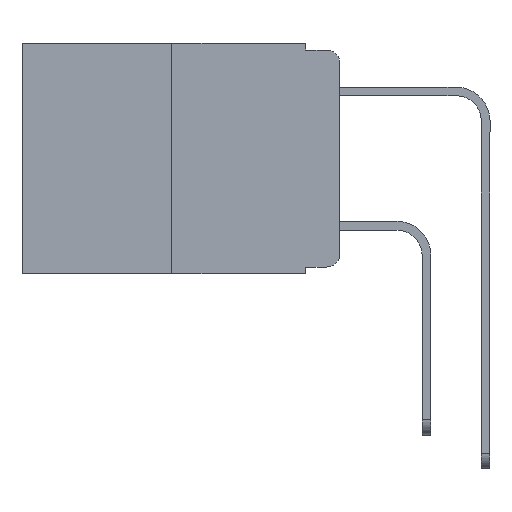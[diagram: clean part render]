
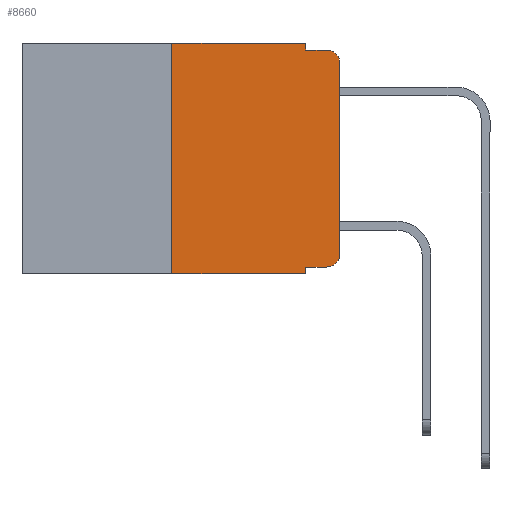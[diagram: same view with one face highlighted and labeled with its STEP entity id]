
A CAD part, left-side view. The second image highlights one B-rep face of the part: STEP entity #8660.
In plain terms, the highlighted planar face has unit normal (-1, 0, 0).
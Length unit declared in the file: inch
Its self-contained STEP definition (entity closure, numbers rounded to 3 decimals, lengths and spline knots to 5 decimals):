
#470 = CARTESIAN_POINT ( 'NONE',  ( 0., 0.25, -0.343 ) ) ;
#684 = EDGE_CURVE ( 'NONE', #8205, #2565, #3473, .T. ) ;
#721 = ORIENTED_EDGE ( 'NONE', *, *, #5792, .T. ) ;
#991 = CARTESIAN_POINT ( 'NONE',  ( 0., 0.02, -0.313 ) ) ;
#1325 = CARTESIAN_POINT ( 'NONE',  ( 0., 0.02, -0.333 ) ) ;
#1469 = CARTESIAN_POINT ( 'NONE',  ( 0., 0.051, -0.01 ) ) ;
#1771 = DIRECTION ( 'NONE',  ( 0., -1., 0. ) ) ;
#1795 = VERTEX_POINT ( 'NONE', #5593 ) ;
#1982 = DIRECTION ( 'NONE',  ( 0., 0., -1. ) ) ;
#2019 = CARTESIAN_POINT ( 'NONE',  ( 0., 0.051, -0.333 ) ) ;
#2071 = DIRECTION ( 'NONE',  ( 0., 0., -1. ) ) ;
#2134 = PLANE ( 'NONE',  #7702 ) ;
#2445 = VECTOR ( 'NONE', #9640, 39.37008 ) ;
#2565 = VERTEX_POINT ( 'NONE', #9895 ) ;
#2645 = CARTESIAN_POINT ( 'NONE',  ( 0., 0., 0. ) ) ;
#2825 = AXIS2_PLACEMENT_3D ( 'NONE', #991, #7983, #1982 ) ;
#2948 = CARTESIAN_POINT ( 'NONE',  ( 0., 0.051, 0. ) ) ;
#3001 = CARTESIAN_POINT ( 'NONE',  ( 0., 0.25, 0. ) ) ;
#3167 = CARTESIAN_POINT ( 'NONE',  ( 0., 0.473, 0. ) ) ;
#3342 = EDGE_CURVE ( 'NONE', #6581, #3847, #6236, .T. ) ;
#3381 = VECTOR ( 'NONE', #4839, 39.37008 ) ;
#3427 = CIRCLE ( 'NONE', #2825, 0.02 ) ;
#3468 = CARTESIAN_POINT ( 'NONE',  ( 0., 0.051, -0.343 ) ) ;
#3473 = LINE ( 'NONE', #1469, #11051 ) ;
#3650 = VERTEX_POINT ( 'NONE', #1325 ) ;
#3667 = EDGE_CURVE ( 'NONE', #11853, #3847, #5440, .T. ) ;
#3695 = VECTOR ( 'NONE', #6827, 39.37008 ) ;
#3847 = VERTEX_POINT ( 'NONE', #3468 ) ;
#3857 = CARTESIAN_POINT ( 'NONE',  ( 0., 0.473, 0. ) ) ;
#3896 = VECTOR ( 'NONE', #7410, 39.37008 ) ;
#3997 = DIRECTION ( 'NONE',  ( 0., 0., 1. ) ) ;
#4024 = FACE_OUTER_BOUND ( 'NONE', #6497, .T. ) ;
#4115 = AXIS2_PLACEMENT_3D ( 'NONE', #12008, #12005, #11989 ) ;
#4173 = DIRECTION ( 'NONE',  ( 0., 0., -1. ) ) ;
#4216 = EDGE_CURVE ( 'NONE', #1795, #4227, #9464, .T. ) ;
#4227 = VERTEX_POINT ( 'NONE', #10710 ) ;
#4302 = CARTESIAN_POINT ( 'NONE',  ( 0., 0.25, 0. ) ) ;
#4498 = ORIENTED_EDGE ( 'NONE', *, *, #11613, .F. ) ;
#4792 = CARTESIAN_POINT ( 'NONE',  ( 0., 0.051, -0.333 ) ) ;
#4839 = DIRECTION ( 'NONE',  ( 0., -1., 0. ) ) ;
#5440 = LINE ( 'NONE', #7324, #2445 ) ;
#5535 = EDGE_CURVE ( 'NONE', #11853, #10641, #12525, .T. ) ;
#5593 = CARTESIAN_POINT ( 'NONE',  ( 0., 0., -0.313 ) ) ;
#5792 = EDGE_CURVE ( 'NONE', #4227, #2565, #11491, .T. ) ;
#6236 = LINE ( 'NONE', #7432, #3896 ) ;
#6245 = ORIENTED_EDGE ( 'NONE', *, *, #684, .F. ) ;
#6497 = EDGE_LOOP ( 'NONE', ( #7029, #721, #6245, #4498, #12639, #8747, #10451, #9523, #11330, #8424 ) ) ;
#6581 = VERTEX_POINT ( 'NONE', #2019 ) ;
#6658 = LINE ( 'NONE', #4792, #3695 ) ;
#6827 = DIRECTION ( 'NONE',  ( 0., -1., 0. ) ) ;
#6981 = LINE ( 'NONE', #3857, #3381 ) ;
#7029 = ORIENTED_EDGE ( 'NONE', *, *, #4216, .T. ) ;
#7324 = CARTESIAN_POINT ( 'NONE',  ( 0., 0.473, -0.343 ) ) ;
#7410 = DIRECTION ( 'NONE',  ( 0., 0., -1. ) ) ;
#7415 = CARTESIAN_POINT ( 'NONE',  ( 0., 0.051, -0.01 ) ) ;
#7432 = CARTESIAN_POINT ( 'NONE',  ( 0., 0.051, 0. ) ) ;
#7702 = AXIS2_PLACEMENT_3D ( 'NONE', #3167, #10120, #4173 ) ;
#7918 = EDGE_CURVE ( 'NONE', #3650, #1795, #3427, .T. ) ;
#7983 = DIRECTION ( 'NONE',  ( -1., 0., 0. ) ) ;
#8069 = CARTESIAN_POINT ( 'NONE',  ( 0., 0.051, 0. ) ) ;
#8205 = VERTEX_POINT ( 'NONE', #7415 ) ;
#8424 = ORIENTED_EDGE ( 'NONE', *, *, #7918, .T. ) ;
#8589 = DIRECTION ( 'NONE',  ( 0., 0., 1. ) ) ;
#8660 = ADVANCED_FACE ( 'NONE', ( #4024 ), #2134, .F. ) ;
#8747 = ORIENTED_EDGE ( 'NONE', *, *, #5535, .F. ) ;
#8989 = LINE ( 'NONE', #8069, #11252 ) ;
#9464 = LINE ( 'NONE', #2645, #12007 ) ;
#9523 = ORIENTED_EDGE ( 'NONE', *, *, #3342, .F. ) ;
#9585 = EDGE_CURVE ( 'NONE', #6581, #3650, #6658, .T. ) ;
#9607 = EDGE_CURVE ( 'NONE', #10641, #11546, #6981, .T. ) ;
#9640 = DIRECTION ( 'NONE',  ( 0., -1., 0. ) ) ;
#9895 = CARTESIAN_POINT ( 'NONE',  ( 0., 0.02, -0.01 ) ) ;
#10021 = VECTOR ( 'NONE', #8589, 39.37008 ) ;
#10120 = DIRECTION ( 'NONE',  ( 1., 0., 0. ) ) ;
#10451 = ORIENTED_EDGE ( 'NONE', *, *, #3667, .T. ) ;
#10641 = VERTEX_POINT ( 'NONE', #4302 ) ;
#10710 = CARTESIAN_POINT ( 'NONE',  ( 0., 0., -0.03 ) ) ;
#11051 = VECTOR ( 'NONE', #1771, 39.37008 ) ;
#11252 = VECTOR ( 'NONE', #2071, 39.37008 ) ;
#11330 = ORIENTED_EDGE ( 'NONE', *, *, #9585, .T. ) ;
#11491 = CIRCLE ( 'NONE', #4115, 0.02 ) ;
#11546 = VERTEX_POINT ( 'NONE', #2948 ) ;
#11613 = EDGE_CURVE ( 'NONE', #11546, #8205, #8989, .T. ) ;
#11853 = VERTEX_POINT ( 'NONE', #470 ) ;
#11989 = DIRECTION ( 'NONE',  ( 0., 0., -1. ) ) ;
#12005 = DIRECTION ( 'NONE',  ( -1., 0., 0. ) ) ;
#12007 = VECTOR ( 'NONE', #3997, 39.37008 ) ;
#12008 = CARTESIAN_POINT ( 'NONE',  ( 0., 0.02, -0.03 ) ) ;
#12525 = LINE ( 'NONE', #3001, #10021 ) ;
#12639 = ORIENTED_EDGE ( 'NONE', *, *, #9607, .F. ) ;
